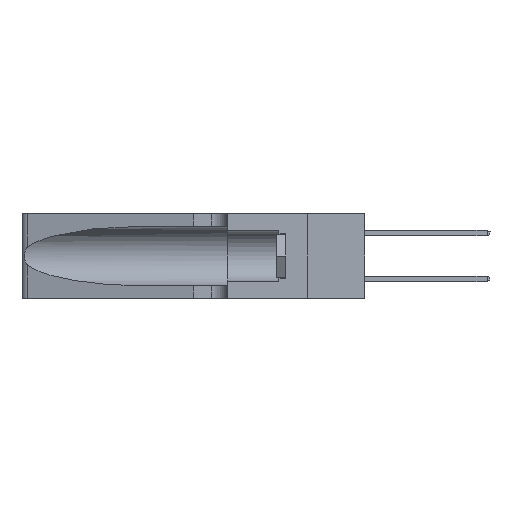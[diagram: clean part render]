
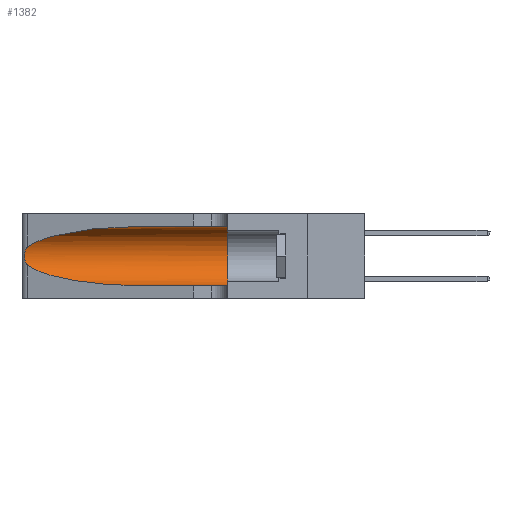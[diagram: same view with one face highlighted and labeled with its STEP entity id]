
A CAD part, left-side view. The second image highlights one B-rep face of the part: STEP entity #1382.
In plain terms, the highlighted cylindrical face has radius 3.308 mm (diameter 6.617 mm), a partial arc.
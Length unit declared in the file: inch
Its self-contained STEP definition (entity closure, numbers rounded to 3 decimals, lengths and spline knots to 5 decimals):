
#474 = EDGE_CURVE ( 'NONE', #12941, #25226, #24205, .T. ) ;
#781 = VERTEX_POINT ( 'NONE', #26183 ) ;
#1382 = ADVANCED_FACE ( 'NONE', ( #9809 ), #24797, .F. ) ;
#1648 = EDGE_CURVE ( 'NONE', #5811, #781, #25840, .T. ) ;
#1722 = DIRECTION ( 'NONE',  ( 0., 0., 1. ) ) ;
#1916 =( BOUNDED_CURVE ( )  B_SPLINE_CURVE ( 3, ( #9634, #21870, #17918, #5571 ),
 .UNSPECIFIED., .F., .F. ) 
 B_SPLINE_CURVE_WITH_KNOTS ( ( 4, 4 ),
 ( 3.44316, 4.71239 ),
 .UNSPECIFIED. ) 
 CURVE ( )  GEOMETRIC_REPRESENTATION_ITEM ( )  RATIONAL_B_SPLINE_CURVE ( ( 1., 0.87, 0.87, 1. ) ) 
 REPRESENTATION_ITEM ( '' )  );
#2082 = CARTESIAN_POINT ( 'NONE',  ( 0.25856, 1.23593, 0.16098 ) ) ;
#2473 = EDGE_LOOP ( 'NONE', ( #18624, #17300, #10886, #24704, #24798, #12013 ) ) ;
#3632 = VERTEX_POINT ( 'NONE', #17279 ) ;
#4181 = DIRECTION ( 'NONE',  ( 0., -1., 0. ) ) ;
#4247 = CARTESIAN_POINT ( 'NONE',  ( 0.25639, 1.23186, 0.15144 ) ) ;
#5267 = EDGE_CURVE ( 'NONE', #3632, #12941, #1916, .T. ) ;
#5404 = CARTESIAN_POINT ( 'NONE',  ( 0.25487, 1.22718, 0.22369 ) ) ;
#5467 = CARTESIAN_POINT ( 'NONE',  ( 0.1305, 0.72297, 0.31525 ) ) ;
#5562 = CARTESIAN_POINT ( 'NONE',  ( 0.18966, 0.96281, 0.31525 ) ) ;
#5571 = CARTESIAN_POINT ( 'NONE',  ( 0.1305, 0.72297, 0.05475 ) ) ;
#5656 = CARTESIAN_POINT ( 'NONE',  ( 0.2373, 1.15595, 0.28018 ) ) ;
#5757 = VERTEX_POINT ( 'NONE', #19297 ) ;
#5811 = VERTEX_POINT ( 'NONE', #25550 ) ;
#6046 = CARTESIAN_POINT ( 'NONE',  ( 0.1305, 1.61858, 0.05475 ) ) ;
#6238 = CARTESIAN_POINT ( 'NONE',  ( 0.25487, 1.22718, 0.22369 ) ) ;
#6323 = CARTESIAN_POINT ( 'NONE',  ( 0.25487, 1.22718, 0.14631 ) ) ;
#7417 = AXIS2_PLACEMENT_3D ( 'NONE', #26357, #14225, #1722 ) ;
#7682 = DIRECTION ( 'NONE',  ( 0., -1., 0. ) ) ;
#8316 = CARTESIAN_POINT ( 'NONE',  ( 0.25639, 1.23184, 0.21858 ) ) ;
#9634 = CARTESIAN_POINT ( 'NONE',  ( 0.25487, 1.22718, 0.14631 ) ) ;
#9809 = FACE_OUTER_BOUND ( 'NONE', #2473, .T. ) ;
#10400 = CARTESIAN_POINT ( 'NONE',  ( 0.25854, 1.2359, 0.20912 ) ) ;
#10647 = EDGE_CURVE ( 'NONE', #781, #3632, #19168, .T. ) ;
#10886 = ORIENTED_EDGE ( 'NONE', *, *, #5267, .T. ) ;
#11265 = LINE ( 'NONE', #26628, #26253 ) ;
#12013 = ORIENTED_EDGE ( 'NONE', *, *, #22827, .F. ) ;
#12484 = CARTESIAN_POINT ( 'NONE',  ( 0.26075, 1.23896, 0.19203 ) ) ;
#12941 = VERTEX_POINT ( 'NONE', #14028 ) ;
#14028 = CARTESIAN_POINT ( 'NONE',  ( 0.1305, 0.72297, 0.05475 ) ) ;
#14225 = DIRECTION ( 'NONE',  ( 0., 1., 0. ) ) ;
#14569 = CARTESIAN_POINT ( 'NONE',  ( 0.26017, 1.23833, 0.17102 ) ) ;
#15970 = CIRCLE ( 'NONE', #7417, 0.13025 ) ;
#16636 = CARTESIAN_POINT ( 'NONE',  ( 0.25789, 1.23486, 0.15765 ) ) ;
#17279 = CARTESIAN_POINT ( 'NONE',  ( 0.25487, 1.22718, 0.14631 ) ) ;
#17300 = ORIENTED_EDGE ( 'NONE', *, *, #10647, .T. ) ;
#17918 = CARTESIAN_POINT ( 'NONE',  ( 0.18966, 0.96281, 0.05475 ) ) ;
#18603 = AXIS2_PLACEMENT_3D ( 'NONE', #24867, #23747, #23599 ) ;
#18624 = ORIENTED_EDGE ( 'NONE', *, *, #1648, .T. ) ;
#18649 = CARTESIAN_POINT ( 'NONE',  ( 0.25555, 1.22993, 0.14849 ) ) ;
#18824 = CARTESIAN_POINT ( 'NONE',  ( 0.1305, 0.35, 0.05475 ) ) ;
#18839 = VECTOR ( 'NONE', #7682, 39.37008 ) ;
#19168 = B_SPLINE_CURVE_WITH_KNOTS ( 'NONE', 3,
 ( #6238, #20607, #8316, #22619, #10400, #24640, #12484, #26689, #14569, #2082, #16636, #4247, #18649, #6323 ),
 .UNSPECIFIED., .F., .F.,
 ( 4, 2, 2, 2, 2, 2, 4 ),
 ( 0., 0.00027, 0.00053, 0.00107, 0.0016, 0.00187, 0.00214 ),
 .UNSPECIFIED. ) ;
#19297 = CARTESIAN_POINT ( 'NONE',  ( 0.1305, 0.35, 0.31525 ) ) ;
#20547 = EDGE_CURVE ( 'NONE', #5757, #25226, #15970, .T. ) ;
#20607 = CARTESIAN_POINT ( 'NONE',  ( 0.25555, 1.22994, 0.2215 ) ) ;
#21870 = CARTESIAN_POINT ( 'NONE',  ( 0.2373, 1.15595, 0.08982 ) ) ;
#22619 = CARTESIAN_POINT ( 'NONE',  ( 0.25787, 1.23484, 0.2124 ) ) ;
#22827 = EDGE_CURVE ( 'NONE', #5811, #5757, #11265, .T. ) ;
#23599 = DIRECTION ( 'NONE',  ( 0., 0., -1. ) ) ;
#23747 = DIRECTION ( 'NONE',  ( 0., -1., 0. ) ) ;
#24205 = LINE ( 'NONE', #6046, #18839 ) ;
#24640 = CARTESIAN_POINT ( 'NONE',  ( 0.26018, 1.23835, 0.19895 ) ) ;
#24704 = ORIENTED_EDGE ( 'NONE', *, *, #474, .T. ) ;
#24797 = CYLINDRICAL_SURFACE ( 'NONE', #18603, 0.13025 ) ;
#24798 = ORIENTED_EDGE ( 'NONE', *, *, #20547, .F. ) ;
#24867 = CARTESIAN_POINT ( 'NONE',  ( 0.1305, 1.61858, 0.185 ) ) ;
#25226 = VERTEX_POINT ( 'NONE', #18824 ) ;
#25550 = CARTESIAN_POINT ( 'NONE',  ( 0.1305, 0.72297, 0.31525 ) ) ;
#25840 =( BOUNDED_CURVE ( )  B_SPLINE_CURVE ( 3, ( #5467, #5562, #5656, #5404 ),
 .UNSPECIFIED., .F., .T. ) 
 B_SPLINE_CURVE_WITH_KNOTS ( ( 4, 4 ),
 ( 1.5708, 2.84003 ),
 .UNSPECIFIED. ) 
 CURVE ( )  GEOMETRIC_REPRESENTATION_ITEM ( )  RATIONAL_B_SPLINE_CURVE ( ( 1., 0.87, 0.87, 1. ) ) 
 REPRESENTATION_ITEM ( '' )  );
#26183 = CARTESIAN_POINT ( 'NONE',  ( 0.25487, 1.22718, 0.22369 ) ) ;
#26253 = VECTOR ( 'NONE', #4181, 39.37008 ) ;
#26357 = CARTESIAN_POINT ( 'NONE',  ( 0.1305, 0.35, 0.185 ) ) ;
#26628 = CARTESIAN_POINT ( 'NONE',  ( 0.1305, 1.61858, 0.31525 ) ) ;
#26689 = CARTESIAN_POINT ( 'NONE',  ( 0.26075, 1.23896, 0.178 ) ) ;
